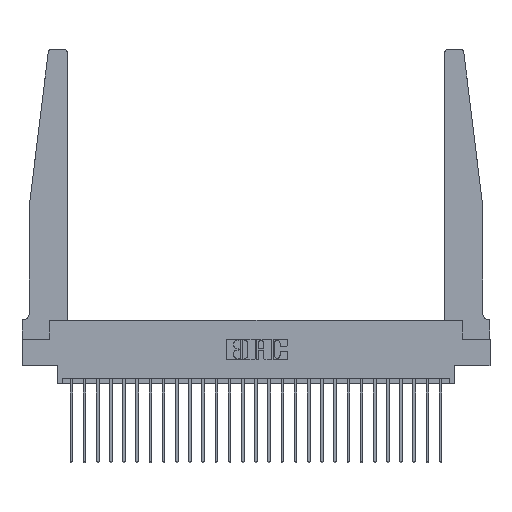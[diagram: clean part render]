
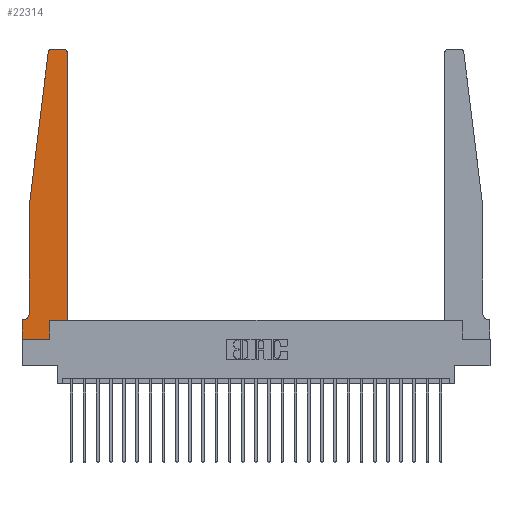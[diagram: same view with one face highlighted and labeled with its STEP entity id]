
A CAD part, top view. The second image highlights one B-rep face of the part: STEP entity #22314.
In plain terms, the highlighted planar face has unit normal (0, 0, 1).
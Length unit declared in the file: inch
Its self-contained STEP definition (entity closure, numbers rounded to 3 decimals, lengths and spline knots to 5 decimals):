
#160 = DIRECTION ( 'NONE',  ( 1., 0., 0. ) ) ;
#452 = VERTEX_POINT ( 'NONE', #25047 ) ;
#977 = AXIS2_PLACEMENT_3D ( 'NONE', #7920, #21781, #9918 ) ;
#1178 = LINE ( 'NONE', #14096, #11136 ) ;
#1596 = CARTESIAN_POINT ( 'NONE',  ( 0.065, 0.1875, 0.37 ) ) ;
#2016 = ORIENTED_EDGE ( 'NONE', *, *, #23603, .T. ) ;
#2041 = LINE ( 'NONE', #6206, #16651 ) ;
#2216 = DIRECTION ( 'NONE',  ( 0., -1., 0. ) ) ;
#2328 = ORIENTED_EDGE ( 'NONE', *, *, #16683, .T. ) ;
#2394 = PLANE ( 'NONE',  #18079 ) ;
#2732 = LINE ( 'NONE', #1596, #8662 ) ;
#3390 = VECTOR ( 'NONE', #9049, 39.37008 ) ;
#3484 = DIRECTION ( 'NONE',  ( -0.122, -0.992, 0. ) ) ;
#3544 = DIRECTION ( 'NONE',  ( 1., 0., 0. ) ) ;
#4234 = VECTOR ( 'NONE', #7634, 39.37008 ) ;
#4907 = AXIS2_PLACEMENT_3D ( 'NONE', #19640, #7745, #21618 ) ;
#5490 = DIRECTION ( 'NONE',  ( -1., 0., 0. ) ) ;
#5510 = EDGE_CURVE ( 'NONE', #18386, #452, #23853, .T. ) ;
#6008 = LINE ( 'NONE', #22944, #11306 ) ;
#6018 = EDGE_CURVE ( 'NONE', #14049, #9205, #2732, .T. ) ;
#6020 = VECTOR ( 'NONE', #3484, 39.37008 ) ;
#6077 = ORIENTED_EDGE ( 'NONE', *, *, #13511, .T. ) ;
#6206 = CARTESIAN_POINT ( 'NONE',  ( 0., 0., 0.37 ) ) ;
#6398 = CARTESIAN_POINT ( 'NONE',  ( 0., 0.1875, 0.37 ) ) ;
#6691 = EDGE_CURVE ( 'NONE', #12417, #18386, #21249, .T. ) ;
#7201 = EDGE_CURVE ( 'NONE', #13527, #23251, #6008, .T. ) ;
#7304 = ORIENTED_EDGE ( 'NONE', *, *, #14496, .T. ) ;
#7634 = DIRECTION ( 'NONE',  ( 0., -1., 0. ) ) ;
#7745 = DIRECTION ( 'NONE',  ( 0., 0., 1. ) ) ;
#7920 = CARTESIAN_POINT ( 'NONE',  ( 0.27653, 2.72, 0.37 ) ) ;
#8148 = VERTEX_POINT ( 'NONE', #24085 ) ;
#8408 = DIRECTION ( 'NONE',  ( 0., 0., 1. ) ) ;
#8662 = VECTOR ( 'NONE', #5490, 39.37008 ) ;
#8955 = VERTEX_POINT ( 'NONE', #20536 ) ;
#9049 = DIRECTION ( 'NONE',  ( 0., 1., 0. ) ) ;
#9088 = DIRECTION ( 'NONE',  ( -1., 0., 0. ) ) ;
#9205 = VERTEX_POINT ( 'NONE', #11255 ) ;
#9499 = ORIENTED_EDGE ( 'NONE', *, *, #6691, .T. ) ;
#9918 = DIRECTION ( 'NONE',  ( 1., 0., 0. ) ) ;
#10070 = VERTEX_POINT ( 'NONE', #14243 ) ;
#10797 = LINE ( 'NONE', #17555, #4234 ) ;
#11039 = VERTEX_POINT ( 'NONE', #21057 ) ;
#11111 = CIRCLE ( 'NONE', #4907, 0.03 ) ;
#11136 = VECTOR ( 'NONE', #16118, 39.37008 ) ;
#11186 = DIRECTION ( 'NONE',  ( 0., 0., -1. ) ) ;
#11248 = LINE ( 'NONE', #17978, #15917 ) ;
#11255 = CARTESIAN_POINT ( 'NONE',  ( 0., 0.1875, 0.37 ) ) ;
#11306 = VECTOR ( 'NONE', #9088, 39.37008 ) ;
#11312 = LINE ( 'NONE', #15415, #6020 ) ;
#11330 = VECTOR ( 'NONE', #3544, 39.37008 ) ;
#11353 = EDGE_CURVE ( 'NONE', #8955, #11039, #1178, .T. ) ;
#11366 = ORIENTED_EDGE ( 'NONE', *, *, #6018, .T. ) ;
#11671 = ORIENTED_EDGE ( 'NONE', *, *, #11856, .T. ) ;
#11856 = EDGE_CURVE ( 'NONE', #11039, #13527, #11111, .T. ) ;
#12417 = VERTEX_POINT ( 'NONE', #19114 ) ;
#12871 = EDGE_LOOP ( 'NONE', ( #13818, #7304, #2016, #21885, #21258, #11366, #6077, #9499, #24611, #2328, #17596, #11671 ) ) ;
#13154 = EDGE_CURVE ( 'NONE', #8148, #14049, #24626, .T. ) ;
#13511 = EDGE_CURVE ( 'NONE', #9205, #12417, #2041, .T. ) ;
#13527 = VERTEX_POINT ( 'NONE', #24023 ) ;
#13540 = FACE_OUTER_BOUND ( 'NONE', #12871, .T. ) ;
#13818 = ORIENTED_EDGE ( 'NONE', *, *, #7201, .T. ) ;
#14049 = VERTEX_POINT ( 'NONE', #18205 ) ;
#14096 = CARTESIAN_POINT ( 'NONE',  ( 0.425, 0.18, 0.37 ) ) ;
#14243 = CARTESIAN_POINT ( 'NONE',  ( 0.24675, 2.72367, 0.37 ) ) ;
#14496 = EDGE_CURVE ( 'NONE', #23251, #10070, #21859, .T. ) ;
#14521 = CARTESIAN_POINT ( 'NONE',  ( 0.2605, 0., 0.37 ) ) ;
#15415 = CARTESIAN_POINT ( 'NONE',  ( 0.065, 1.25, 0.37 ) ) ;
#15470 = CARTESIAN_POINT ( 'NONE',  ( 0., 0., 0.37 ) ) ;
#15917 = VECTOR ( 'NONE', #160, 39.37008 ) ;
#16118 = DIRECTION ( 'NONE',  ( 0., 1., 0. ) ) ;
#16651 = VECTOR ( 'NONE', #2216, 39.37008 ) ;
#16683 = EDGE_CURVE ( 'NONE', #452, #8955, #11248, .T. ) ;
#17555 = CARTESIAN_POINT ( 'NONE',  ( 0.065, 1.25, 0.37 ) ) ;
#17596 = ORIENTED_EDGE ( 'NONE', *, *, #11353, .T. ) ;
#17978 = CARTESIAN_POINT ( 'NONE',  ( 0.425, 0.18, 0.37 ) ) ;
#18079 = AXIS2_PLACEMENT_3D ( 'NONE', #6398, #8408, #22276 ) ;
#18205 = CARTESIAN_POINT ( 'NONE',  ( 0.015, 0.1875, 0.37 ) ) ;
#18386 = VERTEX_POINT ( 'NONE', #14521 ) ;
#18965 = CARTESIAN_POINT ( 'NONE',  ( 0.2605, 0.18, 0.37 ) ) ;
#19114 = CARTESIAN_POINT ( 'NONE',  ( 0., 0., 0.37 ) ) ;
#19185 = EDGE_CURVE ( 'NONE', #21513, #8148, #10797, .T. ) ;
#19640 = CARTESIAN_POINT ( 'NONE',  ( 0.395, 2.72, 0.37 ) ) ;
#20536 = CARTESIAN_POINT ( 'NONE',  ( 0.425, 0.18, 0.37 ) ) ;
#21057 = CARTESIAN_POINT ( 'NONE',  ( 0.425, 2.72, 0.37 ) ) ;
#21249 = LINE ( 'NONE', #15470, #11330 ) ;
#21258 = ORIENTED_EDGE ( 'NONE', *, *, #13154, .T. ) ;
#21513 = VERTEX_POINT ( 'NONE', #25535 ) ;
#21618 = DIRECTION ( 'NONE',  ( 1., 0., 0. ) ) ;
#21781 = DIRECTION ( 'NONE',  ( 0., 0., 1. ) ) ;
#21859 = CIRCLE ( 'NONE', #977, 0.03 ) ;
#21885 = ORIENTED_EDGE ( 'NONE', *, *, #19185, .T. ) ;
#22081 = AXIS2_PLACEMENT_3D ( 'NONE', #23031, #11186, #24978 ) ;
#22276 = DIRECTION ( 'NONE',  ( 1., 0., 0. ) ) ;
#22314 = ADVANCED_FACE ( 'NONE', ( #13540 ), #2394, .T. ) ;
#22944 = CARTESIAN_POINT ( 'NONE',  ( 0.25, 2.75, 0.37 ) ) ;
#23031 = CARTESIAN_POINT ( 'NONE',  ( 0.015, 0.2375, 0.37 ) ) ;
#23251 = VERTEX_POINT ( 'NONE', #24930 ) ;
#23603 = EDGE_CURVE ( 'NONE', #10070, #21513, #11312, .T. ) ;
#23853 = LINE ( 'NONE', #18965, #3390 ) ;
#24023 = CARTESIAN_POINT ( 'NONE',  ( 0.395, 2.75, 0.37 ) ) ;
#24085 = CARTESIAN_POINT ( 'NONE',  ( 0.065, 0.2375, 0.37 ) ) ;
#24611 = ORIENTED_EDGE ( 'NONE', *, *, #5510, .T. ) ;
#24626 = CIRCLE ( 'NONE', #22081, 0.05 ) ;
#24930 = CARTESIAN_POINT ( 'NONE',  ( 0.27653, 2.75, 0.37 ) ) ;
#24978 = DIRECTION ( 'NONE',  ( -1., 0., 0. ) ) ;
#25047 = CARTESIAN_POINT ( 'NONE',  ( 0.2605, 0.18, 0.37 ) ) ;
#25535 = CARTESIAN_POINT ( 'NONE',  ( 0.065, 1.25, 0.37 ) ) ;
